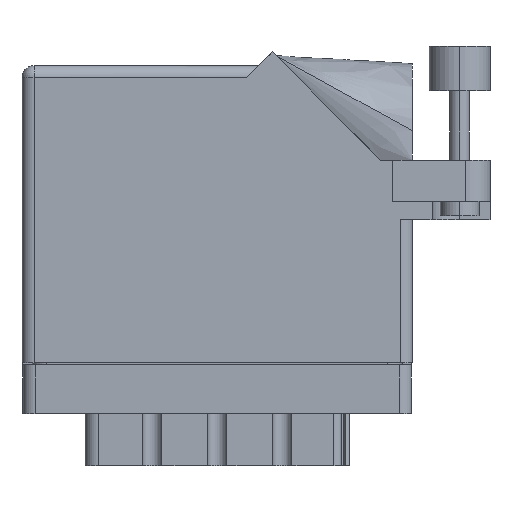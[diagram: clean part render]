
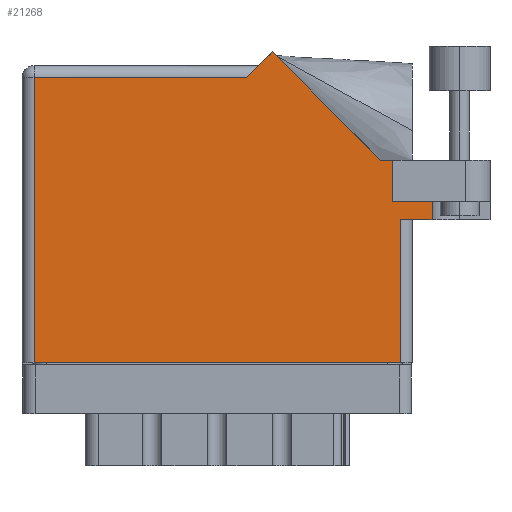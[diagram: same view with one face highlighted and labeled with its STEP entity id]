
A CAD part, front view. The second image highlights one B-rep face of the part: STEP entity #21268.
In plain terms, the highlighted face is planar.
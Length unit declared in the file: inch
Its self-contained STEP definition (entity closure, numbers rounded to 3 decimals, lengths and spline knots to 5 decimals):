
#62 = CARTESIAN_POINT ( 'NONE',  ( 0.062, 0., 0. ) ) ;
#180 = CARTESIAN_POINT ( 'NONE',  ( 2.1115, 0.737, 0. ) ) ;
#980 = VECTOR ( 'NONE', #16381, 39.37008 ) ;
#2049 = FACE_OUTER_BOUND ( 'NONE', #30012, .T. ) ;
#2504 = LINE ( 'NONE', #7055, #14968 ) ;
#2813 = ORIENTED_EDGE ( 'NONE', *, *, #27210, .T. ) ;
#3483 = CARTESIAN_POINT ( 'NONE',  ( 1.948, 0., 0. ) ) ;
#3961 = VECTOR ( 'NONE', #22049, 39.37008 ) ;
#4192 = PLANE ( 'NONE',  #15594 ) ;
#4700 = DIRECTION ( 'NONE',  ( -1., 0., 0. ) ) ;
#4777 = EDGE_CURVE ( 'NONE', #7749, #13247, #41556, .T. ) ;
#5022 = LINE ( 'NONE', #8457, #38591 ) ;
#6102 = CARTESIAN_POINT ( 'NONE',  ( 1.217, 1.53, 0. ) ) ;
#6208 = VERTEX_POINT ( 'NONE', #180 ) ;
#6732 = VERTEX_POINT ( 'NONE', #3483 ) ;
#7055 = CARTESIAN_POINT ( 'NONE',  ( 1.84442, 1.044, 0. ) ) ;
#7191 = CARTESIAN_POINT ( 'NONE',  ( 2.01, 0.737, 0. ) ) ;
#7610 = ORIENTED_EDGE ( 'NONE', *, *, #28800, .T. ) ;
#7749 = VERTEX_POINT ( 'NONE', #35274 ) ;
#8114 = VECTOR ( 'NONE', #4700, 39.37008 ) ;
#8192 = EDGE_CURVE ( 'NONE', #9397, #33198, #19113, .T. ) ;
#8457 = CARTESIAN_POINT ( 'NONE',  ( 0., 0., 0. ) ) ;
#8889 = ORIENTED_EDGE ( 'NONE', *, *, #31155, .T. ) ;
#9181 = ORIENTED_EDGE ( 'NONE', *, *, #4777, .T. ) ;
#9397 = VERTEX_POINT ( 'NONE', #20456 ) ;
#11191 = VERTEX_POINT ( 'NONE', #40588 ) ;
#11479 = LINE ( 'NONE', #35591, #980 ) ;
#12546 = LINE ( 'NONE', #7191, #29068 ) ;
#12631 = DIRECTION ( 'NONE',  ( -1., 0., 0. ) ) ;
#13078 = EDGE_CURVE ( 'NONE', #22504, #40498, #11479, .T. ) ;
#13247 = VERTEX_POINT ( 'NONE', #14677 ) ;
#13853 = ORIENTED_EDGE ( 'NONE', *, *, #36957, .T. ) ;
#13891 = CARTESIAN_POINT ( 'NONE',  ( 0., 1.468, 0. ) ) ;
#14677 = CARTESIAN_POINT ( 'NONE',  ( 1.84442, 1.044, 0. ) ) ;
#14943 = LINE ( 'NONE', #6102, #3961 ) ;
#14968 = VECTOR ( 'NONE', #16705, 39.37008 ) ;
#15594 = AXIS2_PLACEMENT_3D ( 'NONE', #33124, #32982, #20271 ) ;
#16381 = DIRECTION ( 'NONE',  ( 1., 0., 0. ) ) ;
#16705 = DIRECTION ( 'NONE',  ( -0.707, 0.707, 0. ) ) ;
#16764 = EDGE_CURVE ( 'NONE', #33198, #17485, #37080, .T. ) ;
#17462 = VECTOR ( 'NONE', #19248, 39.37008 ) ;
#17485 = VERTEX_POINT ( 'NONE', #25472 ) ;
#17732 = EDGE_CURVE ( 'NONE', #6732, #27404, #38069, .T. ) ;
#17930 = EDGE_CURVE ( 'NONE', #11191, #9397, #14943, .T. ) ;
#18088 = DIRECTION ( 'NONE',  ( 1., 0., 0. ) ) ;
#18912 = CARTESIAN_POINT ( 'NONE',  ( 2.1115, 1.16177, 0. ) ) ;
#19113 = LINE ( 'NONE', #13891, #8114 ) ;
#19248 = DIRECTION ( 'NONE',  ( 0., -1., 0. ) ) ;
#20271 = DIRECTION ( 'NONE',  ( -1., 0., 0. ) ) ;
#20456 = CARTESIAN_POINT ( 'NONE',  ( 1.155, 1.468, 0. ) ) ;
#20788 = LINE ( 'NONE', #38414, #21800 ) ;
#21199 = ORIENTED_EDGE ( 'NONE', *, *, #27572, .F. ) ;
#21268 = ADVANCED_FACE ( 'NONE', ( #2049 ), #4192, .F. ) ;
#21454 = ORIENTED_EDGE ( 'NONE', *, *, #17732, .T. ) ;
#21800 = VECTOR ( 'NONE', #32033, 39.37008 ) ;
#22049 = DIRECTION ( 'NONE',  ( -0.707, -0.707, 0. ) ) ;
#22504 = VERTEX_POINT ( 'NONE', #30163 ) ;
#23151 = DIRECTION ( 'NONE',  ( 1., 0., 0. ) ) ;
#23601 = CARTESIAN_POINT ( 'NONE',  ( 2.1115, 0.831, 0. ) ) ;
#23802 = ORIENTED_EDGE ( 'NONE', *, *, #13078, .F. ) ;
#25472 = CARTESIAN_POINT ( 'NONE',  ( 0.062, 0., 0. ) ) ;
#27169 = CARTESIAN_POINT ( 'NONE',  ( 1.948, 0.737, 0. ) ) ;
#27210 = EDGE_CURVE ( 'NONE', #27404, #6208, #12546, .T. ) ;
#27404 = VERTEX_POINT ( 'NONE', #27169 ) ;
#27572 = EDGE_CURVE ( 'NONE', #40498, #6208, #34572, .T. ) ;
#27853 = ORIENTED_EDGE ( 'NONE', *, *, #17930, .T. ) ;
#27869 = CARTESIAN_POINT ( 'NONE',  ( 0.062, 1.468, 0. ) ) ;
#28165 = CARTESIAN_POINT ( 'NONE',  ( 2.41, 1.044, 0. ) ) ;
#28800 = EDGE_CURVE ( 'NONE', #17485, #6732, #5022, .T. ) ;
#29068 = VECTOR ( 'NONE', #23151, 39.37008 ) ;
#29718 = CARTESIAN_POINT ( 'NONE',  ( 1.948, 0.737, 0. ) ) ;
#30012 = EDGE_LOOP ( 'NONE', ( #7610, #21454, #2813, #21199, #23802, #13853, #9181, #8889, #27853, #37717, #40234 ) ) ;
#30163 = CARTESIAN_POINT ( 'NONE',  ( 1.91, 0.831, 0. ) ) ;
#31155 = EDGE_CURVE ( 'NONE', #13247, #11191, #2504, .T. ) ;
#32033 = DIRECTION ( 'NONE',  ( 0., 1., 0. ) ) ;
#32948 = DIRECTION ( 'NONE',  ( 0., 1., 0. ) ) ;
#32982 = DIRECTION ( 'NONE',  ( 0., 0., -1. ) ) ;
#33124 = CARTESIAN_POINT ( 'NONE',  ( 0., 1.53, 0. ) ) ;
#33198 = VERTEX_POINT ( 'NONE', #27869 ) ;
#33542 = VECTOR ( 'NONE', #41237, 39.37008 ) ;
#34518 = VECTOR ( 'NONE', #12631, 39.37008 ) ;
#34572 = LINE ( 'NONE', #18912, #33542 ) ;
#35274 = CARTESIAN_POINT ( 'NONE',  ( 1.91, 1.044, 0. ) ) ;
#35591 = CARTESIAN_POINT ( 'NONE',  ( 1.91, 0.831, 0. ) ) ;
#36957 = EDGE_CURVE ( 'NONE', #22504, #7749, #20788, .T. ) ;
#37049 = VECTOR ( 'NONE', #32948, 39.37008 ) ;
#37080 = LINE ( 'NONE', #62, #17462 ) ;
#37717 = ORIENTED_EDGE ( 'NONE', *, *, #8192, .T. ) ;
#38069 = LINE ( 'NONE', #29718, #37049 ) ;
#38414 = CARTESIAN_POINT ( 'NONE',  ( 1.91, 0.831, 0. ) ) ;
#38591 = VECTOR ( 'NONE', #18088, 39.37008 ) ;
#40234 = ORIENTED_EDGE ( 'NONE', *, *, #16764, .T. ) ;
#40498 = VERTEX_POINT ( 'NONE', #23601 ) ;
#40588 = CARTESIAN_POINT ( 'NONE',  ( 1.28771, 1.60071, 0. ) ) ;
#41237 = DIRECTION ( 'NONE',  ( 0., -1., 0. ) ) ;
#41556 = LINE ( 'NONE', #28165, #34518 ) ;
